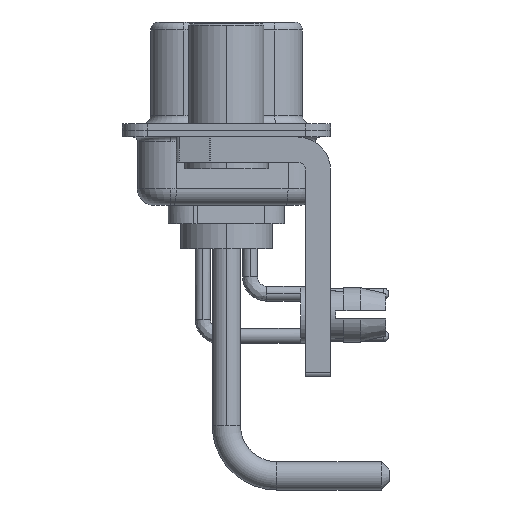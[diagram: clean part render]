
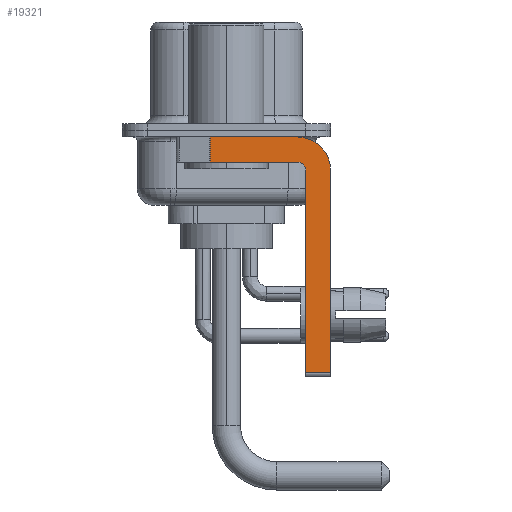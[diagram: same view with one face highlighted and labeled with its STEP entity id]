
A CAD part, left-side view. The second image highlights one B-rep face of the part: STEP entity #19321.
In plain terms, the highlighted planar face has unit normal (-1, 0, 0).
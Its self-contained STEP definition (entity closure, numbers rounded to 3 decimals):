
#365 = VERTEX_POINT ( 'NONE', #17899 ) ;
#558 = CARTESIAN_POINT ( 'NONE',  ( -2.9, -4.25, -2.4 ) ) ;
#782 = AXIS2_PLACEMENT_3D ( 'NONE', #17480, #13135, #15653 ) ;
#832 = DIRECTION ( 'NONE',  ( 1., 0., 0. ) ) ;
#999 = LINE ( 'NONE', #9576, #25813 ) ;
#1435 = EDGE_CURVE ( 'NONE', #8592, #10979, #21309, .T. ) ;
#2550 = VECTOR ( 'NONE', #18159, 1000. ) ;
#2633 = DIRECTION ( 'NONE',  ( 0., 0., -1. ) ) ;
#2954 = PLANE ( 'NONE',  #19154 ) ;
#2969 = EDGE_CURVE ( 'NONE', #4075, #21891, #7957, .T. ) ;
#3146 = ORIENTED_EDGE ( 'NONE', *, *, #6962, .F. ) ;
#3389 = EDGE_CURVE ( 'NONE', #10979, #365, #12890, .T. ) ;
#4075 = VERTEX_POINT ( 'NONE', #20251 ) ;
#4361 = CARTESIAN_POINT ( 'NONE',  ( -2.9, 0.978, -0.4 ) ) ;
#4688 = VERTEX_POINT ( 'NONE', #14708 ) ;
#5065 = EDGE_CURVE ( 'NONE', #19208, #22366, #6092, .T. ) ;
#6092 = LINE ( 'NONE', #23487, #25502 ) ;
#6138 = AXIS2_PLACEMENT_3D ( 'NONE', #6996, #7138, #2633 ) ;
#6588 = CARTESIAN_POINT ( 'NONE',  ( -2.9, -4.75, -14.55 ) ) ;
#6922 = EDGE_CURVE ( 'NONE', #8592, #4688, #7321, .T. ) ;
#6962 = EDGE_CURVE ( 'NONE', #21891, #4688, #27057, .T. ) ;
#6996 = CARTESIAN_POINT ( 'NONE',  ( -2.9, -4.25, -2.4 ) ) ;
#7138 = DIRECTION ( 'NONE',  ( 1., 0., 0. ) ) ;
#7321 = LINE ( 'NONE', #15868, #10937 ) ;
#7957 = CIRCLE ( 'NONE', #6138, 2. ) ;
#8592 = VERTEX_POINT ( 'NONE', #6588 ) ;
#9576 = CARTESIAN_POINT ( 'NONE',  ( -2.9, 3., -0.4 ) ) ;
#9603 = CARTESIAN_POINT ( 'NONE',  ( -2.9, -4.25, -1.9 ) ) ;
#10937 = VECTOR ( 'NONE', #13356, 1000. ) ;
#10979 = VERTEX_POINT ( 'NONE', #15109 ) ;
#11721 = CARTESIAN_POINT ( 'NONE',  ( -2.9, 0.978, -1.9 ) ) ;
#12890 = CIRCLE ( 'NONE', #782, 0.5 ) ;
#13135 = DIRECTION ( 'NONE',  ( -1., 0., 0. ) ) ;
#13356 = DIRECTION ( 'NONE',  ( 0., -1., 0. ) ) ;
#14051 = VECTOR ( 'NONE', #27199, 1000. ) ;
#14258 = ORIENTED_EDGE ( 'NONE', *, *, #2969, .F. ) ;
#14708 = CARTESIAN_POINT ( 'NONE',  ( -2.9, -6.25, -14.55 ) ) ;
#15109 = CARTESIAN_POINT ( 'NONE',  ( -2.9, -4.75, -2.4 ) ) ;
#15653 = DIRECTION ( 'NONE',  ( 0., 0., 1. ) ) ;
#15868 = CARTESIAN_POINT ( 'NONE',  ( -2.9, -4.25, -14.55 ) ) ;
#15880 = ORIENTED_EDGE ( 'NONE', *, *, #5065, .T. ) ;
#16549 = CARTESIAN_POINT ( 'NONE',  ( -2.9, -6.25, -2.4 ) ) ;
#16613 = DIRECTION ( 'NONE',  ( 0., 0., -1. ) ) ;
#16735 = EDGE_CURVE ( 'NONE', #19208, #4075, #999, .T. ) ;
#17480 = CARTESIAN_POINT ( 'NONE',  ( -2.9, -4.25, -2.4 ) ) ;
#17683 = DIRECTION ( 'NONE',  ( 0., 0., -1. ) ) ;
#17899 = CARTESIAN_POINT ( 'NONE',  ( -2.9, -4.25, -1.9 ) ) ;
#18159 = DIRECTION ( 'NONE',  ( 0., 1., 0. ) ) ;
#19154 = AXIS2_PLACEMENT_3D ( 'NONE', #558, #832, #17683 ) ;
#19208 = VERTEX_POINT ( 'NONE', #4361 ) ;
#19321 = ADVANCED_FACE ( 'NONE', ( #22180 ), #2954, .F. ) ;
#19606 = ORIENTED_EDGE ( 'NONE', *, *, #1435, .F. ) ;
#19959 = DIRECTION ( 'NONE',  ( 0., -1., 0. ) ) ;
#19990 = LINE ( 'NONE', #9603, #2550 ) ;
#20201 = ORIENTED_EDGE ( 'NONE', *, *, #27033, .F. ) ;
#20251 = CARTESIAN_POINT ( 'NONE',  ( -2.9, -4.25, -0.4 ) ) ;
#21309 = LINE ( 'NONE', #21443, #22969 ) ;
#21443 = CARTESIAN_POINT ( 'NONE',  ( -2.9, -4.75, -14.8 ) ) ;
#21891 = VERTEX_POINT ( 'NONE', #24516 ) ;
#22180 = FACE_OUTER_BOUND ( 'NONE', #26912, .T. ) ;
#22366 = VERTEX_POINT ( 'NONE', #11721 ) ;
#22969 = VECTOR ( 'NONE', #25238, 1000. ) ;
#23487 = CARTESIAN_POINT ( 'NONE',  ( -2.9, 0.978, -1.9 ) ) ;
#24163 = ORIENTED_EDGE ( 'NONE', *, *, #3389, .F. ) ;
#24516 = CARTESIAN_POINT ( 'NONE',  ( -2.9, -6.25, -2.4 ) ) ;
#25229 = ORIENTED_EDGE ( 'NONE', *, *, #6922, .T. ) ;
#25238 = DIRECTION ( 'NONE',  ( 0., 0., 1. ) ) ;
#25502 = VECTOR ( 'NONE', #16613, 1000. ) ;
#25813 = VECTOR ( 'NONE', #19959, 1000. ) ;
#26571 = ORIENTED_EDGE ( 'NONE', *, *, #16735, .F. ) ;
#26912 = EDGE_LOOP ( 'NONE', ( #26571, #15880, #20201, #24163, #19606, #25229, #3146, #14258 ) ) ;
#27033 = EDGE_CURVE ( 'NONE', #365, #22366, #19990, .T. ) ;
#27057 = LINE ( 'NONE', #16549, #14051 ) ;
#27199 = DIRECTION ( 'NONE',  ( 0., 0., -1. ) ) ;
